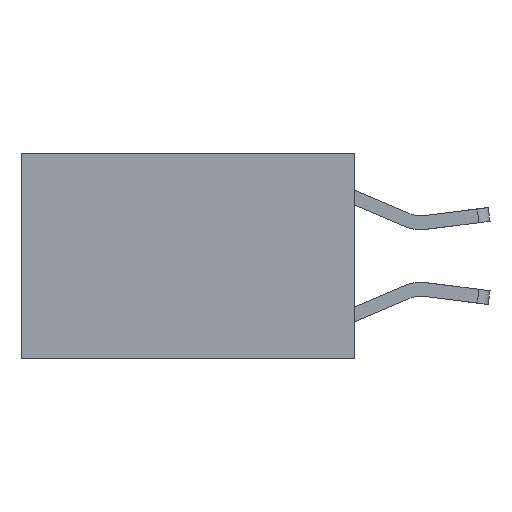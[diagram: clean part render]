
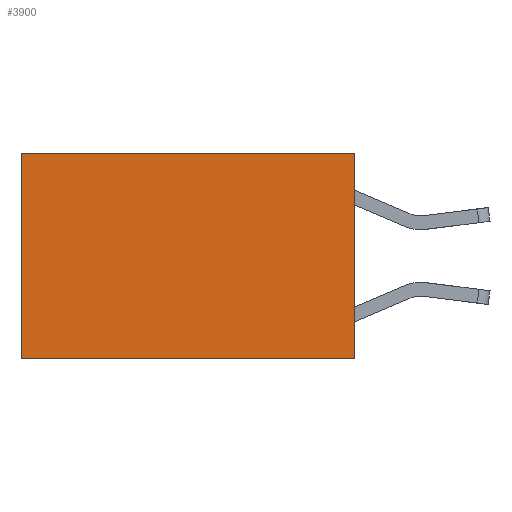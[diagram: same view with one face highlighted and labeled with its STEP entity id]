
A CAD part, left-side view. The second image highlights one B-rep face of the part: STEP entity #3900.
In plain terms, the highlighted planar face has unit normal (-1, 0, 0).
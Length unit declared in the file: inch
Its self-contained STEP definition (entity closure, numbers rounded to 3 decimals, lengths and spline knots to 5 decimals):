
#381 = EDGE_CURVE ( 'NONE', #1363, #7552, #4038, .T. ) ;
#451 = CARTESIAN_POINT ( 'NONE',  ( 0.2625, 0., -0.37 ) ) ;
#1056 = EDGE_CURVE ( 'NONE', #8242, #9049, #11728, .T. ) ;
#1173 = EDGE_CURVE ( 'NONE', #9049, #7552, #6885, .T. ) ;
#1363 = VERTEX_POINT ( 'NONE', #11431 ) ;
#1419 = VECTOR ( 'NONE', #10608, 39.37008 ) ;
#1425 = LINE ( 'NONE', #5669, #9552 ) ;
#1851 = VECTOR ( 'NONE', #7822, 39.37008 ) ;
#3900 = ADVANCED_FACE ( 'NONE', ( #6765 ), #5820, .F. ) ;
#4008 = EDGE_LOOP ( 'NONE', ( #12739, #4594, #6045, #10661 ) ) ;
#4038 = LINE ( 'NONE', #11323, #4881 ) ;
#4392 = EDGE_CURVE ( 'NONE', #8242, #1363, #1425, .T. ) ;
#4594 = ORIENTED_EDGE ( 'NONE', *, *, #1173, .F. ) ;
#4881 = VECTOR ( 'NONE', #13443, 39.37008 ) ;
#5669 = CARTESIAN_POINT ( 'NONE',  ( 0.2625, 0., 0. ) ) ;
#5796 = CARTESIAN_POINT ( 'NONE',  ( 0.2625, 0., 0. ) ) ;
#5820 = PLANE ( 'NONE',  #9317 ) ;
#6045 = ORIENTED_EDGE ( 'NONE', *, *, #1056, .F. ) ;
#6765 = FACE_OUTER_BOUND ( 'NONE', #4008, .T. ) ;
#6885 = LINE ( 'NONE', #451, #1851 ) ;
#7552 = VERTEX_POINT ( 'NONE', #11809 ) ;
#7767 = CARTESIAN_POINT ( 'NONE',  ( 0.2625, 0., 0. ) ) ;
#7822 = DIRECTION ( 'NONE',  ( 0., 1., 0. ) ) ;
#8242 = VERTEX_POINT ( 'NONE', #5796 ) ;
#8510 = CARTESIAN_POINT ( 'NONE',  ( 0.2625, 0., 0. ) ) ;
#9049 = VERTEX_POINT ( 'NONE', #10901 ) ;
#9317 = AXIS2_PLACEMENT_3D ( 'NONE', #7767, #12006, #9956 ) ;
#9552 = VECTOR ( 'NONE', #11927, 39.37008 ) ;
#9956 = DIRECTION ( 'NONE',  ( 0., 0., -1. ) ) ;
#10608 = DIRECTION ( 'NONE',  ( 0., 0., -1. ) ) ;
#10661 = ORIENTED_EDGE ( 'NONE', *, *, #4392, .T. ) ;
#10901 = CARTESIAN_POINT ( 'NONE',  ( 0.2625, 0., -0.37 ) ) ;
#11323 = CARTESIAN_POINT ( 'NONE',  ( 0.2625, 0.6, 0. ) ) ;
#11431 = CARTESIAN_POINT ( 'NONE',  ( 0.2625, 0.6, 0. ) ) ;
#11728 = LINE ( 'NONE', #8510, #1419 ) ;
#11809 = CARTESIAN_POINT ( 'NONE',  ( 0.2625, 0.6, -0.37 ) ) ;
#11927 = DIRECTION ( 'NONE',  ( 0., 1., 0. ) ) ;
#12006 = DIRECTION ( 'NONE',  ( 1., 0., 0. ) ) ;
#12739 = ORIENTED_EDGE ( 'NONE', *, *, #381, .T. ) ;
#13443 = DIRECTION ( 'NONE',  ( 0., 0., -1. ) ) ;
